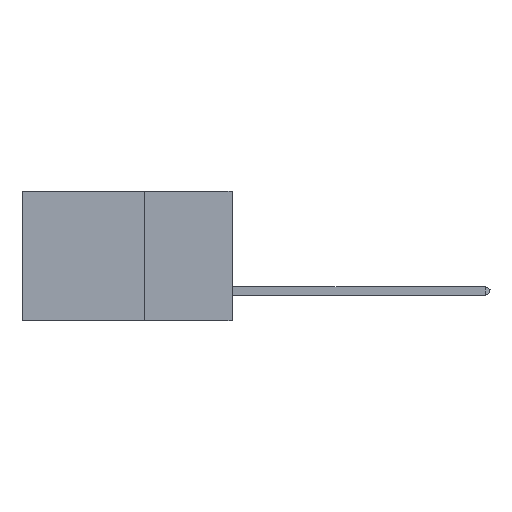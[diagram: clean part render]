
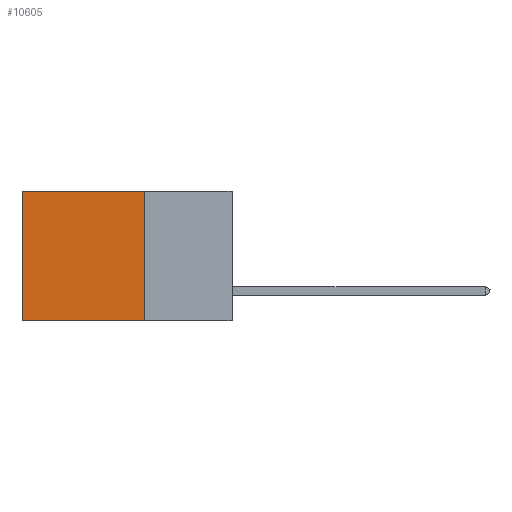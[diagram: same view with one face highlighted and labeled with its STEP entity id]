
A CAD part, left-side view. The second image highlights one B-rep face of the part: STEP entity #10605.
In plain terms, the highlighted planar face has unit normal (-1, 0, 0).
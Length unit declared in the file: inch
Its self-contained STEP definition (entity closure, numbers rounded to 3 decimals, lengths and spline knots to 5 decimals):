
#692 = VERTEX_POINT ( 'NONE', #18690 ) ;
#955 = CARTESIAN_POINT ( 'NONE',  ( 0.2875, 0.25, 0. ) ) ;
#2426 = CARTESIAN_POINT ( 'NONE',  ( 0.2875, 0.25, 0. ) ) ;
#2565 = DIRECTION ( 'NONE',  ( 0., 0., -1. ) ) ;
#2582 = ORIENTED_EDGE ( 'NONE', *, *, #41836, .F. ) ;
#3128 = EDGE_CURVE ( 'NONE', #29326, #11275, #37447, .T. ) ;
#3509 = FACE_OUTER_BOUND ( 'NONE', #36549, .T. ) ;
#3839 = CARTESIAN_POINT ( 'NONE',  ( 0.2875, 0.25, 0. ) ) ;
#5556 = DIRECTION ( 'NONE',  ( 0., 1., 0. ) ) ;
#5675 = DIRECTION ( 'NONE',  ( 1., 0., 0. ) ) ;
#5948 = VERTEX_POINT ( 'NONE', #955 ) ;
#6732 = EDGE_CURVE ( 'NONE', #5948, #29326, #34145, .T. ) ;
#8918 = PLANE ( 'NONE',  #25829 ) ;
#9948 = VECTOR ( 'NONE', #5556, 39.37008 ) ;
#10146 = ORIENTED_EDGE ( 'NONE', *, *, #6732, .T. ) ;
#10325 = LINE ( 'NONE', #23491, #35064 ) ;
#10605 = ADVANCED_FACE ( 'NONE', ( #3509 ), #8918, .F. ) ;
#11275 = VERTEX_POINT ( 'NONE', #19538 ) ;
#13681 = CARTESIAN_POINT ( 'NONE',  ( 0.2875, 0.6, 0. ) ) ;
#14639 = CARTESIAN_POINT ( 'NONE',  ( 0.2875, 0.6, 0. ) ) ;
#18690 = CARTESIAN_POINT ( 'NONE',  ( 0.2875, 0.25, -0.37 ) ) ;
#19443 = DIRECTION ( 'NONE',  ( 0., 1., 0. ) ) ;
#19538 = CARTESIAN_POINT ( 'NONE',  ( 0.2875, 0.6, -0.37 ) ) ;
#19876 = VECTOR ( 'NONE', #19443, 39.37008 ) ;
#22249 = ORIENTED_EDGE ( 'NONE', *, *, #3128, .T. ) ;
#23272 = VECTOR ( 'NONE', #37144, 39.37008 ) ;
#23491 = CARTESIAN_POINT ( 'NONE',  ( 0.2875, 0.25, 0. ) ) ;
#25131 = EDGE_CURVE ( 'NONE', #5948, #692, #10325, .T. ) ;
#25829 = AXIS2_PLACEMENT_3D ( 'NONE', #2426, #5675, #2565 ) ;
#26862 = DIRECTION ( 'NONE',  ( 0., 0., -1. ) ) ;
#26961 = LINE ( 'NONE', #32134, #19876 ) ;
#29326 = VERTEX_POINT ( 'NONE', #13681 ) ;
#32134 = CARTESIAN_POINT ( 'NONE',  ( 0.2875, 0.25, -0.37 ) ) ;
#34145 = LINE ( 'NONE', #3839, #9948 ) ;
#35064 = VECTOR ( 'NONE', #26862, 39.37008 ) ;
#36549 = EDGE_LOOP ( 'NONE', ( #22249, #2582, #38476, #10146 ) ) ;
#37144 = DIRECTION ( 'NONE',  ( 0., 0., -1. ) ) ;
#37447 = LINE ( 'NONE', #14639, #23272 ) ;
#38476 = ORIENTED_EDGE ( 'NONE', *, *, #25131, .F. ) ;
#41836 = EDGE_CURVE ( 'NONE', #692, #11275, #26961, .T. ) ;
